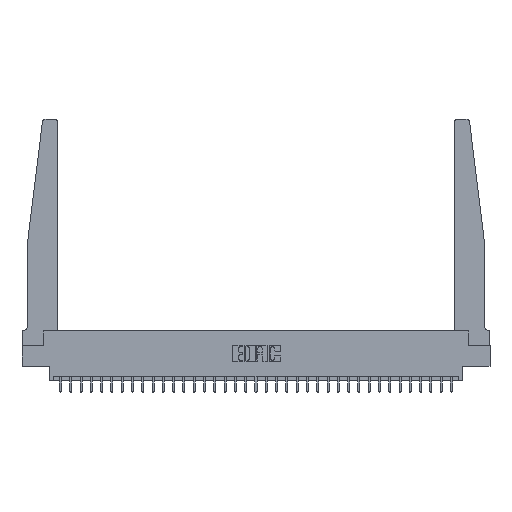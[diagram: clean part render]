
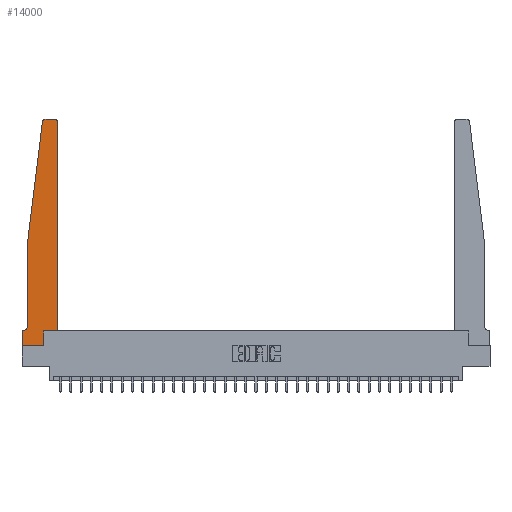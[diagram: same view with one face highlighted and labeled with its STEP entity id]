
A CAD part, top view. The second image highlights one B-rep face of the part: STEP entity #14000.
In plain terms, the highlighted planar face has unit normal (0, 0, 1).
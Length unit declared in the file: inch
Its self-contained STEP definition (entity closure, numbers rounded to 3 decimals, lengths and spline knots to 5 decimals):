
#783 = LINE ( 'NONE', #20079, #14807 ) ;
#821 = CARTESIAN_POINT ( 'NONE',  ( 0.24675, 2.72367, 0.37 ) ) ;
#984 = VERTEX_POINT ( 'NONE', #18869 ) ;
#1095 = VERTEX_POINT ( 'NONE', #16353 ) ;
#1611 = CARTESIAN_POINT ( 'NONE',  ( 0.065, 1.25, 0.37 ) ) ;
#1638 = CIRCLE ( 'NONE', #23360, 0.03 ) ;
#1877 = CARTESIAN_POINT ( 'NONE',  ( 0., 0., 0.37 ) ) ;
#2823 = DIRECTION ( 'NONE',  ( -1., 0., 0. ) ) ;
#2825 = ORIENTED_EDGE ( 'NONE', *, *, #20902, .T. ) ;
#3290 = VECTOR ( 'NONE', #20929, 39.37008 ) ;
#3947 = DIRECTION ( 'NONE',  ( 1., 0., 0. ) ) ;
#4077 = VECTOR ( 'NONE', #21306, 39.37008 ) ;
#4844 = LINE ( 'NONE', #16557, #4077 ) ;
#5134 = CARTESIAN_POINT ( 'NONE',  ( 0., 0.1875, 0.37 ) ) ;
#5575 = CARTESIAN_POINT ( 'NONE',  ( 0., 0., 0.37 ) ) ;
#5614 = EDGE_CURVE ( 'NONE', #1095, #8879, #20775, .T. ) ;
#5959 = DIRECTION ( 'NONE',  ( -1., 0., 0. ) ) ;
#5995 = DIRECTION ( 'NONE',  ( 1., 0., 0. ) ) ;
#6096 = VERTEX_POINT ( 'NONE', #21976 ) ;
#6205 = ORIENTED_EDGE ( 'NONE', *, *, #27621, .T. ) ;
#6593 = DIRECTION ( 'NONE',  ( 0., 0., 1. ) ) ;
#7600 = EDGE_CURVE ( 'NONE', #24748, #11934, #10255, .T. ) ;
#7737 = CARTESIAN_POINT ( 'NONE',  ( 0.065, 1.25, 0.37 ) ) ;
#7811 = ORIENTED_EDGE ( 'NONE', *, *, #7600, .T. ) ;
#7949 = LINE ( 'NONE', #5575, #28926 ) ;
#8176 = VERTEX_POINT ( 'NONE', #16983 ) ;
#8348 = DIRECTION ( 'NONE',  ( -0.122, -0.992, 0. ) ) ;
#8879 = VERTEX_POINT ( 'NONE', #9439 ) ;
#8907 = EDGE_LOOP ( 'NONE', ( #7811, #6205, #21122, #19357, #19813, #28042, #30915, #27737, #19834, #22496, #23648, #2825 ) ) ;
#8934 = AXIS2_PLACEMENT_3D ( 'NONE', #9933, #17204, #17039 ) ;
#9439 = CARTESIAN_POINT ( 'NONE',  ( 0.2605, 0.18, 0.37 ) ) ;
#9837 = EDGE_CURVE ( 'NONE', #31162, #8176, #18704, .T. ) ;
#9933 = CARTESIAN_POINT ( 'NONE',  ( 0.27653, 2.72, 0.37 ) ) ;
#9959 = VECTOR ( 'NONE', #2823, 39.37008 ) ;
#10191 = DIRECTION ( 'NONE',  ( 0., 0., 1. ) ) ;
#10255 = LINE ( 'NONE', #14999, #9959 ) ;
#11289 = CARTESIAN_POINT ( 'NONE',  ( 0.2605, 0.18, 0.37 ) ) ;
#11814 = VERTEX_POINT ( 'NONE', #15958 ) ;
#11934 = VERTEX_POINT ( 'NONE', #17800 ) ;
#12173 = EDGE_CURVE ( 'NONE', #8176, #6096, #14610, .T. ) ;
#12243 = DIRECTION ( 'NONE',  ( 1., 0., 0. ) ) ;
#12713 = FACE_OUTER_BOUND ( 'NONE', #8907, .T. ) ;
#12796 = LINE ( 'NONE', #7737, #16530 ) ;
#12864 = PLANE ( 'NONE',  #18221 ) ;
#13081 = VECTOR ( 'NONE', #28331, 39.37008 ) ;
#13399 = EDGE_CURVE ( 'NONE', #6096, #984, #4844, .T. ) ;
#14000 = ADVANCED_FACE ( 'NONE', ( #12713 ), #12864, .T. ) ;
#14271 = DIRECTION ( 'NONE',  ( 0., 1., 0. ) ) ;
#14610 = CIRCLE ( 'NONE', #28209, 0.05 ) ;
#14807 = VECTOR ( 'NONE', #5995, 39.37008 ) ;
#14852 = VECTOR ( 'NONE', #3947, 39.37008 ) ;
#14999 = CARTESIAN_POINT ( 'NONE',  ( 0.25, 2.75, 0.37 ) ) ;
#15549 = DIRECTION ( 'NONE',  ( 0., -1., 0. ) ) ;
#15958 = CARTESIAN_POINT ( 'NONE',  ( 0., 0., 0.37 ) ) ;
#16187 = LINE ( 'NONE', #28631, #30093 ) ;
#16353 = CARTESIAN_POINT ( 'NONE',  ( 0.2605, 0., 0.37 ) ) ;
#16530 = VECTOR ( 'NONE', #8348, 39.37008 ) ;
#16557 = CARTESIAN_POINT ( 'NONE',  ( 0.065, 0.1875, 0.37 ) ) ;
#16983 = CARTESIAN_POINT ( 'NONE',  ( 0.065, 0.2375, 0.37 ) ) ;
#17039 = DIRECTION ( 'NONE',  ( 1., 0., 0. ) ) ;
#17204 = DIRECTION ( 'NONE',  ( 0., 0., 1. ) ) ;
#17800 = CARTESIAN_POINT ( 'NONE',  ( 0.27653, 2.75, 0.37 ) ) ;
#17875 = CARTESIAN_POINT ( 'NONE',  ( 0.395, 2.75, 0.37 ) ) ;
#17982 = CARTESIAN_POINT ( 'NONE',  ( 0.015, 0.2375, 0.37 ) ) ;
#18221 = AXIS2_PLACEMENT_3D ( 'NONE', #5134, #10191, #29771 ) ;
#18704 = LINE ( 'NONE', #1611, #13081 ) ;
#18869 = CARTESIAN_POINT ( 'NONE',  ( 0., 0.1875, 0.37 ) ) ;
#19343 = CARTESIAN_POINT ( 'NONE',  ( 0.395, 2.72, 0.37 ) ) ;
#19357 = ORIENTED_EDGE ( 'NONE', *, *, #9837, .T. ) ;
#19813 = ORIENTED_EDGE ( 'NONE', *, *, #12173, .T. ) ;
#19834 = ORIENTED_EDGE ( 'NONE', *, *, #5614, .T. ) ;
#20079 = CARTESIAN_POINT ( 'NONE',  ( 0.425, 0.18, 0.37 ) ) ;
#20775 = LINE ( 'NONE', #11289, #3290 ) ;
#20902 = EDGE_CURVE ( 'NONE', #31027, #24748, #1638, .T. ) ;
#20929 = DIRECTION ( 'NONE',  ( 0., 1., 0. ) ) ;
#20997 = EDGE_CURVE ( 'NONE', #984, #11814, #7949, .T. ) ;
#21037 = VERTEX_POINT ( 'NONE', #821 ) ;
#21122 = ORIENTED_EDGE ( 'NONE', *, *, #25986, .T. ) ;
#21306 = DIRECTION ( 'NONE',  ( -1., 0., 0. ) ) ;
#21321 = EDGE_CURVE ( 'NONE', #8879, #24546, #783, .T. ) ;
#21521 = EDGE_CURVE ( 'NONE', #11814, #1095, #27961, .T. ) ;
#21976 = CARTESIAN_POINT ( 'NONE',  ( 0.015, 0.1875, 0.37 ) ) ;
#22496 = ORIENTED_EDGE ( 'NONE', *, *, #21321, .T. ) ;
#23360 = AXIS2_PLACEMENT_3D ( 'NONE', #19343, #6593, #12243 ) ;
#23648 = ORIENTED_EDGE ( 'NONE', *, *, #25170, .T. ) ;
#24521 = CARTESIAN_POINT ( 'NONE',  ( 0.425, 0.18, 0.37 ) ) ;
#24546 = VERTEX_POINT ( 'NONE', #24521 ) ;
#24748 = VERTEX_POINT ( 'NONE', #17875 ) ;
#25170 = EDGE_CURVE ( 'NONE', #24546, #31027, #16187, .T. ) ;
#25986 = EDGE_CURVE ( 'NONE', #21037, #31162, #12796, .T. ) ;
#27606 = DIRECTION ( 'NONE',  ( 0., 0., -1. ) ) ;
#27621 = EDGE_CURVE ( 'NONE', #11934, #21037, #28596, .T. ) ;
#27737 = ORIENTED_EDGE ( 'NONE', *, *, #21521, .T. ) ;
#27961 = LINE ( 'NONE', #1877, #14852 ) ;
#28042 = ORIENTED_EDGE ( 'NONE', *, *, #13399, .T. ) ;
#28209 = AXIS2_PLACEMENT_3D ( 'NONE', #17982, #27606, #5959 ) ;
#28331 = DIRECTION ( 'NONE',  ( 0., -1., 0. ) ) ;
#28596 = CIRCLE ( 'NONE', #8934, 0.03 ) ;
#28631 = CARTESIAN_POINT ( 'NONE',  ( 0.425, 0.18, 0.37 ) ) ;
#28926 = VECTOR ( 'NONE', #15549, 39.37008 ) ;
#29771 = DIRECTION ( 'NONE',  ( 1., 0., 0. ) ) ;
#29979 = CARTESIAN_POINT ( 'NONE',  ( 0.425, 2.72, 0.37 ) ) ;
#30093 = VECTOR ( 'NONE', #14271, 39.37008 ) ;
#30764 = CARTESIAN_POINT ( 'NONE',  ( 0.065, 1.25, 0.37 ) ) ;
#30915 = ORIENTED_EDGE ( 'NONE', *, *, #20997, .T. ) ;
#31027 = VERTEX_POINT ( 'NONE', #29979 ) ;
#31162 = VERTEX_POINT ( 'NONE', #30764 ) ;
